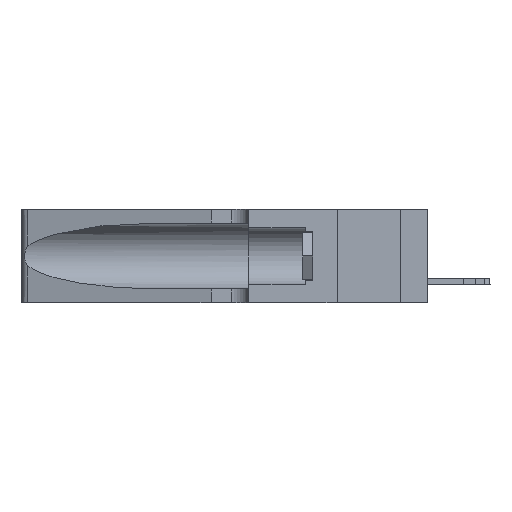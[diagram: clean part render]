
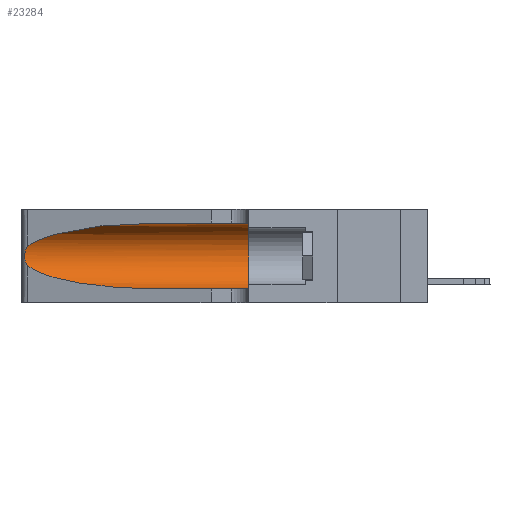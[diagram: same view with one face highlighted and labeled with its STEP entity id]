
A CAD part, left-side view. The second image highlights one B-rep face of the part: STEP entity #23284.
In plain terms, the highlighted cylindrical face has radius 3.308 mm (diameter 6.617 mm), a partial arc.
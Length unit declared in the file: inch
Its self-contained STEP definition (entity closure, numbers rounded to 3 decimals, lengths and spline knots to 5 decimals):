
#17 = CARTESIAN_POINT ( 'NONE',  ( 0.25487, 1.22718, 0.22369 ) ) ;
#246 = DIRECTION ( 'NONE',  ( 0., -1., 0. ) ) ;
#864 = VERTEX_POINT ( 'NONE', #20077 ) ;
#1550 = CARTESIAN_POINT ( 'NONE',  ( 0.1305, 0.72297, 0.05475 ) ) ;
#1626 = DIRECTION ( 'NONE',  ( 0., -1., 0. ) ) ;
#3099 = CARTESIAN_POINT ( 'NONE',  ( 0.26017, 1.23833, 0.17102 ) ) ;
#3360 = CARTESIAN_POINT ( 'NONE',  ( 0.2373, 1.15595, 0.08982 ) ) ;
#3771 =( BOUNDED_CURVE ( )  B_SPLINE_CURVE ( 3, ( #9775, #3360, #13651, #4166 ),
 .UNSPECIFIED., .F., .F. ) 
 B_SPLINE_CURVE_WITH_KNOTS ( ( 4, 4 ),
 ( 3.44316, 4.71239 ),
 .UNSPECIFIED. ) 
 CURVE ( )  GEOMETRIC_REPRESENTATION_ITEM ( )  RATIONAL_B_SPLINE_CURVE ( ( 1., 0.87, 0.87, 1. ) ) 
 REPRESENTATION_ITEM ( '' )  );
#4166 = CARTESIAN_POINT ( 'NONE',  ( 0.1305, 0.72297, 0.05475 ) ) ;
#4237 = ORIENTED_EDGE ( 'NONE', *, *, #40573, .T. ) ;
#4299 = B_SPLINE_CURVE_WITH_KNOTS ( 'NONE', 3,
 ( #17, #15540, #18889, #38147, #6190, #28437, #9387, #31637, #3099, #25388, #34988, #19134, #19760, #32031 ),
 .UNSPECIFIED., .F., .F.,
 ( 4, 2, 2, 2, 2, 2, 4 ),
 ( 0., 0.00027, 0.00053, 0.00107, 0.0016, 0.00187, 0.00214 ),
 .UNSPECIFIED. ) ;
#5703 = EDGE_CURVE ( 'NONE', #864, #11870, #4299, .T. ) ;
#5778 = CARTESIAN_POINT ( 'NONE',  ( 0.1305, 0.35, 0.185 ) ) ;
#6190 = CARTESIAN_POINT ( 'NONE',  ( 0.25854, 1.2359, 0.20912 ) ) ;
#6649 = DIRECTION ( 'NONE',  ( 0., -1., 0. ) ) ;
#6973 = ORIENTED_EDGE ( 'NONE', *, *, #14165, .T. ) ;
#9387 = CARTESIAN_POINT ( 'NONE',  ( 0.26075, 1.23896, 0.19203 ) ) ;
#9775 = CARTESIAN_POINT ( 'NONE',  ( 0.25487, 1.22718, 0.14631 ) ) ;
#9849 = VERTEX_POINT ( 'NONE', #26327 ) ;
#10017 = VECTOR ( 'NONE', #6649, 39.37008 ) ;
#11870 = VERTEX_POINT ( 'NONE', #39408 ) ;
#11965 = CARTESIAN_POINT ( 'NONE',  ( 0.1305, 0.35, 0.31525 ) ) ;
#12549 = CARTESIAN_POINT ( 'NONE',  ( 0.1305, 1.61858, 0.05475 ) ) ;
#12779 = EDGE_LOOP ( 'NONE', ( #34152, #40571, #6973, #4237, #33268, #38593 ) ) ;
#12925 = EDGE_CURVE ( 'NONE', #24300, #9849, #39611, .T. ) ;
#13651 = CARTESIAN_POINT ( 'NONE',  ( 0.18966, 0.96281, 0.05475 ) ) ;
#13809 = CARTESIAN_POINT ( 'NONE',  ( 0.1305, 0.72297, 0.31525 ) ) ;
#14165 = EDGE_CURVE ( 'NONE', #11870, #14820, #3771, .T. ) ;
#14276 = EDGE_CURVE ( 'NONE', #37960, #24300, #30558, .T. ) ;
#14820 = VERTEX_POINT ( 'NONE', #1550 ) ;
#15540 = CARTESIAN_POINT ( 'NONE',  ( 0.25555, 1.22994, 0.2215 ) ) ;
#16569 = DIRECTION ( 'NONE',  ( 0., 0., -1. ) ) ;
#16626 = VECTOR ( 'NONE', #1626, 39.37008 ) ;
#16968 = CARTESIAN_POINT ( 'NONE',  ( 0.1305, 0.72297, 0.31525 ) ) ;
#17111 = CYLINDRICAL_SURFACE ( 'NONE', #25922, 0.13025 ) ;
#18889 = CARTESIAN_POINT ( 'NONE',  ( 0.25639, 1.23184, 0.21858 ) ) ;
#19134 = CARTESIAN_POINT ( 'NONE',  ( 0.25639, 1.23186, 0.15144 ) ) ;
#19760 = CARTESIAN_POINT ( 'NONE',  ( 0.25555, 1.22993, 0.14849 ) ) ;
#20077 = CARTESIAN_POINT ( 'NONE',  ( 0.25487, 1.22718, 0.22369 ) ) ;
#20293 = CARTESIAN_POINT ( 'NONE',  ( 0.1305, 1.61858, 0.31525 ) ) ;
#20322 = CARTESIAN_POINT ( 'NONE',  ( 0.25487, 1.22718, 0.22369 ) ) ;
#23284 = ADVANCED_FACE ( 'NONE', ( #33024 ), #17111, .F. ) ;
#24300 = VERTEX_POINT ( 'NONE', #11965 ) ;
#24971 = DIRECTION ( 'NONE',  ( 0., 0., 1. ) ) ;
#25388 = CARTESIAN_POINT ( 'NONE',  ( 0.25856, 1.23593, 0.16098 ) ) ;
#25922 = AXIS2_PLACEMENT_3D ( 'NONE', #32403, #246, #16569 ) ;
#26327 = CARTESIAN_POINT ( 'NONE',  ( 0.1305, 0.35, 0.05475 ) ) ;
#26920 = LINE ( 'NONE', #12549, #10017 ) ;
#28437 = CARTESIAN_POINT ( 'NONE',  ( 0.26018, 1.23835, 0.19895 ) ) ;
#30525 = EDGE_CURVE ( 'NONE', #37960, #864, #32630, .T. ) ;
#30558 = LINE ( 'NONE', #20293, #16626 ) ;
#31637 = CARTESIAN_POINT ( 'NONE',  ( 0.26075, 1.23896, 0.178 ) ) ;
#32031 = CARTESIAN_POINT ( 'NONE',  ( 0.25487, 1.22718, 0.14631 ) ) ;
#32403 = CARTESIAN_POINT ( 'NONE',  ( 0.1305, 1.61858, 0.185 ) ) ;
#32630 =( BOUNDED_CURVE ( )  B_SPLINE_CURVE ( 3, ( #13809, #35908, #39345, #20322 ),
 .UNSPECIFIED., .F., .T. ) 
 B_SPLINE_CURVE_WITH_KNOTS ( ( 4, 4 ),
 ( 1.5708, 2.84003 ),
 .UNSPECIFIED. ) 
 CURVE ( )  GEOMETRIC_REPRESENTATION_ITEM ( )  RATIONAL_B_SPLINE_CURVE ( ( 1., 0.87, 0.87, 1. ) ) 
 REPRESENTATION_ITEM ( '' )  );
#33024 = FACE_OUTER_BOUND ( 'NONE', #12779, .T. ) ;
#33268 = ORIENTED_EDGE ( 'NONE', *, *, #12925, .F. ) ;
#34008 = DIRECTION ( 'NONE',  ( 0., 1., 0. ) ) ;
#34152 = ORIENTED_EDGE ( 'NONE', *, *, #30525, .T. ) ;
#34988 = CARTESIAN_POINT ( 'NONE',  ( 0.25789, 1.23486, 0.15765 ) ) ;
#35908 = CARTESIAN_POINT ( 'NONE',  ( 0.18966, 0.96281, 0.31525 ) ) ;
#37960 = VERTEX_POINT ( 'NONE', #16968 ) ;
#38147 = CARTESIAN_POINT ( 'NONE',  ( 0.25787, 1.23484, 0.2124 ) ) ;
#38593 = ORIENTED_EDGE ( 'NONE', *, *, #14276, .F. ) ;
#39345 = CARTESIAN_POINT ( 'NONE',  ( 0.2373, 1.15595, 0.28018 ) ) ;
#39408 = CARTESIAN_POINT ( 'NONE',  ( 0.25487, 1.22718, 0.14631 ) ) ;
#39611 = CIRCLE ( 'NONE', #40282, 0.13025 ) ;
#40282 = AXIS2_PLACEMENT_3D ( 'NONE', #5778, #34008, #24971 ) ;
#40571 = ORIENTED_EDGE ( 'NONE', *, *, #5703, .T. ) ;
#40573 = EDGE_CURVE ( 'NONE', #14820, #9849, #26920, .T. ) ;
